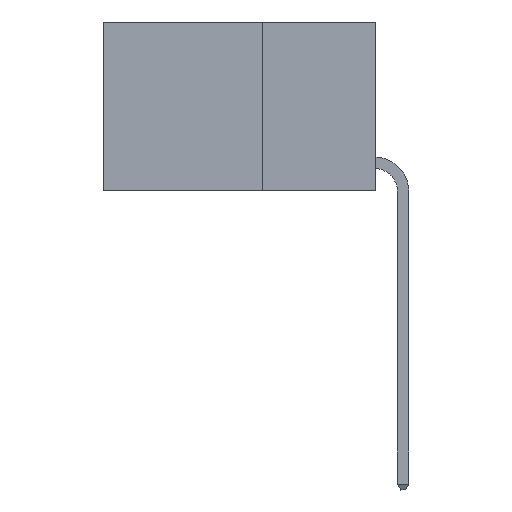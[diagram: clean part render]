
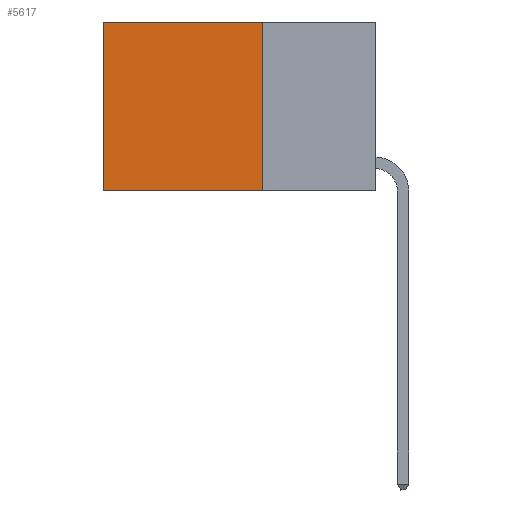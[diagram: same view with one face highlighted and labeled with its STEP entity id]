
A CAD part, left-side view. The second image highlights one B-rep face of the part: STEP entity #5617.
In plain terms, the highlighted planar face has unit normal (-1, 0, 0).
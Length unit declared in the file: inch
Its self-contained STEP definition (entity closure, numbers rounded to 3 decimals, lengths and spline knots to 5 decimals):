
#412 = EDGE_CURVE ( 'NONE', #11753, #4264, #16641, .T. ) ;
#488 = LINE ( 'NONE', #5911, #15452 ) ;
#1207 = VECTOR ( 'NONE', #11363, 39.37008 ) ;
#1528 = ORIENTED_EDGE ( 'NONE', *, *, #8158, .F. ) ;
#2744 = CARTESIAN_POINT ( 'NONE',  ( 0.2625, 0.25, -0.37 ) ) ;
#2975 = LINE ( 'NONE', #12561, #11104 ) ;
#3003 = DIRECTION ( 'NONE',  ( 0., 0., -1. ) ) ;
#3378 = VECTOR ( 'NONE', #3003, 39.37008 ) ;
#3927 = CARTESIAN_POINT ( 'NONE',  ( 0.2625, 0.25, 0. ) ) ;
#4264 = VERTEX_POINT ( 'NONE', #4901 ) ;
#4901 = CARTESIAN_POINT ( 'NONE',  ( 0.2625, 0.6, -0.37 ) ) ;
#5617 = ADVANCED_FACE ( 'NONE', ( #7713 ), #13107, .F. ) ;
#5911 = CARTESIAN_POINT ( 'NONE',  ( 0.2625, 0.6, 0. ) ) ;
#6212 = ORIENTED_EDGE ( 'NONE', *, *, #15162, .T. ) ;
#6388 = ORIENTED_EDGE ( 'NONE', *, *, #412, .F. ) ;
#7611 = VERTEX_POINT ( 'NONE', #12261 ) ;
#7713 = FACE_OUTER_BOUND ( 'NONE', #7752, .T. ) ;
#7752 = EDGE_LOOP ( 'NONE', ( #8071, #6388, #1528, #6212 ) ) ;
#8071 = ORIENTED_EDGE ( 'NONE', *, *, #9490, .T. ) ;
#8158 = EDGE_CURVE ( 'NONE', #7611, #11753, #15051, .T. ) ;
#8403 = DIRECTION ( 'NONE',  ( 0., 1., 0. ) ) ;
#9490 = EDGE_CURVE ( 'NONE', #11655, #4264, #488, .T. ) ;
#11104 = VECTOR ( 'NONE', #8403, 39.37008 ) ;
#11363 = DIRECTION ( 'NONE',  ( 0., 1., 0. ) ) ;
#11655 = VERTEX_POINT ( 'NONE', #14448 ) ;
#11744 = AXIS2_PLACEMENT_3D ( 'NONE', #3927, #12022, #14401 ) ;
#11753 = VERTEX_POINT ( 'NONE', #2744 ) ;
#12022 = DIRECTION ( 'NONE',  ( 1., 0., 0. ) ) ;
#12261 = CARTESIAN_POINT ( 'NONE',  ( 0.2625, 0.25, 0. ) ) ;
#12561 = CARTESIAN_POINT ( 'NONE',  ( 0.2625, 0.25, 0. ) ) ;
#12783 = CARTESIAN_POINT ( 'NONE',  ( 0.2625, 0.25, -0.37 ) ) ;
#13107 = PLANE ( 'NONE',  #11744 ) ;
#14401 = DIRECTION ( 'NONE',  ( 0., 0., -1. ) ) ;
#14448 = CARTESIAN_POINT ( 'NONE',  ( 0.2625, 0.6, 0. ) ) ;
#15051 = LINE ( 'NONE', #16474, #3378 ) ;
#15162 = EDGE_CURVE ( 'NONE', #7611, #11655, #2975, .T. ) ;
#15452 = VECTOR ( 'NONE', #16744, 39.37008 ) ;
#16474 = CARTESIAN_POINT ( 'NONE',  ( 0.2625, 0.25, 0. ) ) ;
#16641 = LINE ( 'NONE', #12783, #1207 ) ;
#16744 = DIRECTION ( 'NONE',  ( 0., 0., -1. ) ) ;
